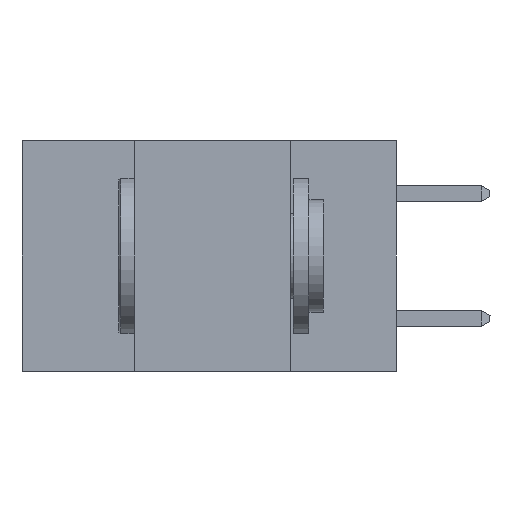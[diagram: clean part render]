
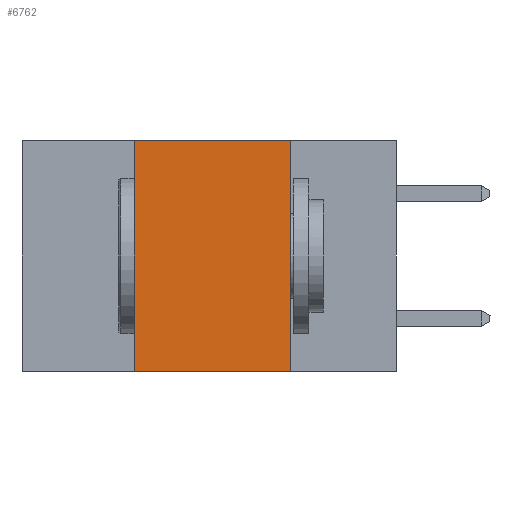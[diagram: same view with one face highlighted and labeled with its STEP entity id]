
A CAD part, left-side view. The second image highlights one B-rep face of the part: STEP entity #6762.
In plain terms, the highlighted planar face has unit normal (-1, 0, 0).
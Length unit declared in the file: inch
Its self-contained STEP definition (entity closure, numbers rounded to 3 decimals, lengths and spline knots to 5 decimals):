
#30 = AXIS2_PLACEMENT_3D ( 'NONE', #2037, #4938, #11250 ) ;
#503 = VECTOR ( 'NONE', #5637, 39.37008 ) ;
#1279 = ORIENTED_EDGE ( 'NONE', *, *, #5152, .T. ) ;
#1512 = ORIENTED_EDGE ( 'NONE', *, *, #10896, .F. ) ;
#1595 = ORIENTED_EDGE ( 'NONE', *, *, #8566, .F. ) ;
#2037 = CARTESIAN_POINT ( 'NONE',  ( 0., 0.6, 0. ) ) ;
#2388 = CARTESIAN_POINT ( 'NONE',  ( 0., 0.6, -0.37 ) ) ;
#2782 = EDGE_LOOP ( 'NONE', ( #1595, #6169, #1512, #1279 ) ) ;
#3000 = LINE ( 'NONE', #10145, #503 ) ;
#3109 = CARTESIAN_POINT ( 'NONE',  ( 0., 0.42, 0. ) ) ;
#3358 = DIRECTION ( 'NONE',  ( 0., -1., 0. ) ) ;
#3366 = VECTOR ( 'NONE', #3358, 39.37008 ) ;
#3444 = CARTESIAN_POINT ( 'NONE',  ( 0., 0.42, -0.37 ) ) ;
#3558 = LINE ( 'NONE', #10840, #8790 ) ;
#3662 = VERTEX_POINT ( 'NONE', #11351 ) ;
#4938 = DIRECTION ( 'NONE',  ( 1., 0., 0. ) ) ;
#5152 = EDGE_CURVE ( 'NONE', #5200, #8969, #10705, .T. ) ;
#5200 = VERTEX_POINT ( 'NONE', #10790 ) ;
#5637 = DIRECTION ( 'NONE',  ( 0., 0., -1. ) ) ;
#6169 = ORIENTED_EDGE ( 'NONE', *, *, #10313, .F. ) ;
#6762 = ADVANCED_FACE ( 'NONE', ( #8116 ), #10374, .F. ) ;
#7255 = DIRECTION ( 'NONE',  ( 0., -1., 0. ) ) ;
#8116 = FACE_OUTER_BOUND ( 'NONE', #2782, .T. ) ;
#8566 = EDGE_CURVE ( 'NONE', #3662, #8969, #3000, .T. ) ;
#8790 = VECTOR ( 'NONE', #7255, 39.37008 ) ;
#8969 = VERTEX_POINT ( 'NONE', #10676 ) ;
#9198 = VECTOR ( 'NONE', #11634, 39.37008 ) ;
#10145 = CARTESIAN_POINT ( 'NONE',  ( 0., 0.17, -0.37 ) ) ;
#10313 = EDGE_CURVE ( 'NONE', #10712, #3662, #3558, .T. ) ;
#10374 = PLANE ( 'NONE',  #30 ) ;
#10676 = CARTESIAN_POINT ( 'NONE',  ( 0., 0.17, -0.37 ) ) ;
#10705 = LINE ( 'NONE', #2388, #3366 ) ;
#10712 = VERTEX_POINT ( 'NONE', #3109 ) ;
#10790 = CARTESIAN_POINT ( 'NONE',  ( 0., 0.42, -0.37 ) ) ;
#10840 = CARTESIAN_POINT ( 'NONE',  ( 0., 0.6, 0. ) ) ;
#10896 = EDGE_CURVE ( 'NONE', #5200, #10712, #11513, .T. ) ;
#11250 = DIRECTION ( 'NONE',  ( 0., 0., -1. ) ) ;
#11351 = CARTESIAN_POINT ( 'NONE',  ( 0., 0.17, 0. ) ) ;
#11513 = LINE ( 'NONE', #3444, #9198 ) ;
#11634 = DIRECTION ( 'NONE',  ( 0., 0., 1. ) ) ;
